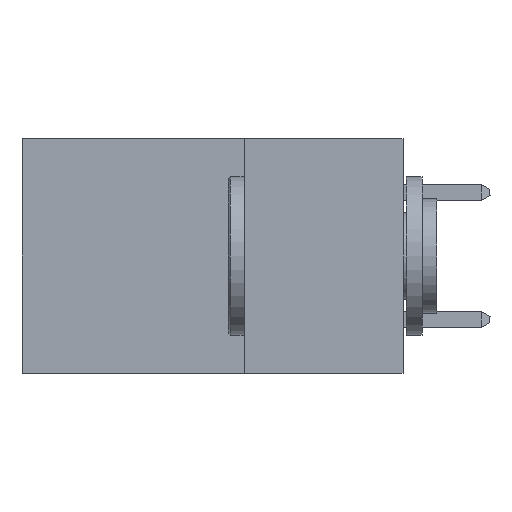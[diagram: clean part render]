
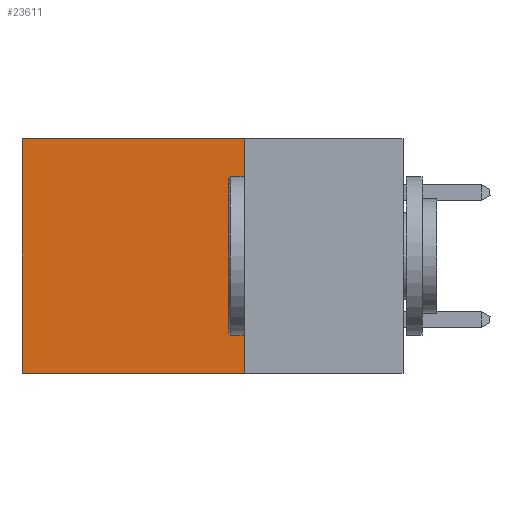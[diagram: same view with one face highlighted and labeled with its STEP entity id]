
A CAD part, left-side view. The second image highlights one B-rep face of the part: STEP entity #23611.
In plain terms, the highlighted planar face has unit normal (-1, 0, 0).
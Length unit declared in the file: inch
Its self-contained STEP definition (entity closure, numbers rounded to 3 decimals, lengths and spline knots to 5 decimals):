
#751 = LINE ( 'NONE', #35536, #15314 ) ;
#1205 = AXIS2_PLACEMENT_3D ( 'NONE', #2597, #16167, #26736 ) ;
#1547 = DIRECTION ( 'NONE',  ( 0., 0., -1. ) ) ;
#2597 = CARTESIAN_POINT ( 'NONE',  ( 0.2875, 0.25, 0. ) ) ;
#4621 = LINE ( 'NONE', #35975, #34373 ) ;
#6323 = DIRECTION ( 'NONE',  ( 0., 1., 0. ) ) ;
#9086 = LINE ( 'NONE', #30490, #22567 ) ;
#10909 = VERTEX_POINT ( 'NONE', #33864 ) ;
#11230 = LINE ( 'NONE', #38981, #23082 ) ;
#12202 = ORIENTED_EDGE ( 'NONE', *, *, #27018, .T. ) ;
#12419 = FACE_OUTER_BOUND ( 'NONE', #18903, .T. ) ;
#15314 = VECTOR ( 'NONE', #17855, 39.37008 ) ;
#16167 = DIRECTION ( 'NONE',  ( 1., 0., 0. ) ) ;
#17834 = CARTESIAN_POINT ( 'NONE',  ( 0.2875, 0.6, -0.37 ) ) ;
#17855 = DIRECTION ( 'NONE',  ( 0., 1., 0. ) ) ;
#18903 = EDGE_LOOP ( 'NONE', ( #12202, #36399, #43239, #25883 ) ) ;
#19055 = EDGE_CURVE ( 'NONE', #22652, #32369, #11230, .T. ) ;
#22567 = VECTOR ( 'NONE', #6323, 39.37008 ) ;
#22652 = VERTEX_POINT ( 'NONE', #38300 ) ;
#23082 = VECTOR ( 'NONE', #25237, 39.37008 ) ;
#23611 = ADVANCED_FACE ( 'NONE', ( #12419 ), #40473, .F. ) ;
#25237 = DIRECTION ( 'NONE',  ( 0., 0., -1. ) ) ;
#25883 = ORIENTED_EDGE ( 'NONE', *, *, #31564, .T. ) ;
#26509 = VERTEX_POINT ( 'NONE', #17834 ) ;
#26736 = DIRECTION ( 'NONE',  ( 0., 0., -1. ) ) ;
#27018 = EDGE_CURVE ( 'NONE', #10909, #26509, #4621, .T. ) ;
#30490 = CARTESIAN_POINT ( 'NONE',  ( 0.2875, 0.25, 0. ) ) ;
#31564 = EDGE_CURVE ( 'NONE', #22652, #10909, #9086, .T. ) ;
#32369 = VERTEX_POINT ( 'NONE', #33779 ) ;
#33779 = CARTESIAN_POINT ( 'NONE',  ( 0.2875, 0.25, -0.37 ) ) ;
#33864 = CARTESIAN_POINT ( 'NONE',  ( 0.2875, 0.6, 0. ) ) ;
#34373 = VECTOR ( 'NONE', #1547, 39.37008 ) ;
#34441 = EDGE_CURVE ( 'NONE', #32369, #26509, #751, .T. ) ;
#35536 = CARTESIAN_POINT ( 'NONE',  ( 0.2875, 0.25, -0.37 ) ) ;
#35975 = CARTESIAN_POINT ( 'NONE',  ( 0.2875, 0.6, 0. ) ) ;
#36399 = ORIENTED_EDGE ( 'NONE', *, *, #34441, .F. ) ;
#38300 = CARTESIAN_POINT ( 'NONE',  ( 0.2875, 0.25, 0. ) ) ;
#38981 = CARTESIAN_POINT ( 'NONE',  ( 0.2875, 0.25, 0. ) ) ;
#40473 = PLANE ( 'NONE',  #1205 ) ;
#43239 = ORIENTED_EDGE ( 'NONE', *, *, #19055, .F. ) ;
